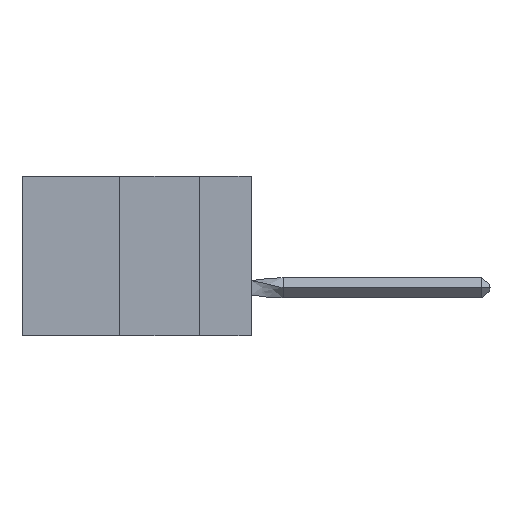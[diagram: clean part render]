
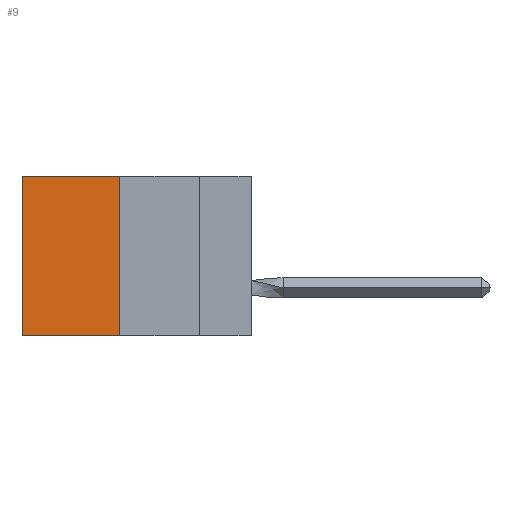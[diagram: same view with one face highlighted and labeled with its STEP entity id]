
A CAD part, left-side view. The second image highlights one B-rep face of the part: STEP entity #9.
In plain terms, the highlighted planar face has unit normal (-1, 0, 0).
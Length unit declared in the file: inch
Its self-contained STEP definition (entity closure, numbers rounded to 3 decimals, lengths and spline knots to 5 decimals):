
#9 = ADVANCED_FACE ( 'NONE', ( #1995 ), #11821, .F. ) ;
#97 = VERTEX_POINT ( 'NONE', #4743 ) ;
#1810 = CARTESIAN_POINT ( 'NONE',  ( 0.305, 0.413, -0.5 ) ) ;
#1995 = FACE_OUTER_BOUND ( 'NONE', #10964, .T. ) ;
#2162 = AXIS2_PLACEMENT_3D ( 'NONE', #10183, #5823, #2902 ) ;
#2425 = VECTOR ( 'NONE', #12045, 39.37008 ) ;
#2432 = ORIENTED_EDGE ( 'NONE', *, *, #2916, .F. ) ;
#2772 = VECTOR ( 'NONE', #9825, 39.37008 ) ;
#2902 = DIRECTION ( 'NONE',  ( 0., 0., -1. ) ) ;
#2916 = EDGE_CURVE ( 'NONE', #9484, #15254, #4434, .T. ) ;
#3051 = CARTESIAN_POINT ( 'NONE',  ( 0.305, 0.413, 0. ) ) ;
#4003 = CARTESIAN_POINT ( 'NONE',  ( 0.305, 0.413, -0.5 ) ) ;
#4434 = LINE ( 'NONE', #6071, #2425 ) ;
#4503 = CARTESIAN_POINT ( 'NONE',  ( 0.305, 0.413, 0. ) ) ;
#4509 = ORIENTED_EDGE ( 'NONE', *, *, #4709, .T. ) ;
#4709 = EDGE_CURVE ( 'NONE', #15734, #97, #6680, .T. ) ;
#4743 = CARTESIAN_POINT ( 'NONE',  ( 0.305, 0.72, -0.5 ) ) ;
#5823 = DIRECTION ( 'NONE',  ( 1., 0., 0. ) ) ;
#5915 = DIRECTION ( 'NONE',  ( 0., 1., 0. ) ) ;
#6071 = CARTESIAN_POINT ( 'NONE',  ( 0.305, 0.413, -0.5 ) ) ;
#6227 = VECTOR ( 'NONE', #6794, 39.37008 ) ;
#6680 = LINE ( 'NONE', #11145, #6227 ) ;
#6794 = DIRECTION ( 'NONE',  ( 0., 0., -1. ) ) ;
#9398 = EDGE_CURVE ( 'NONE', #9484, #15734, #13157, .T. ) ;
#9484 = VERTEX_POINT ( 'NONE', #3051 ) ;
#9825 = DIRECTION ( 'NONE',  ( 0., 1., 0. ) ) ;
#10153 = CARTESIAN_POINT ( 'NONE',  ( 0.305, 0.72, 0. ) ) ;
#10183 = CARTESIAN_POINT ( 'NONE',  ( 0.305, 0.413, -0.5 ) ) ;
#10964 = EDGE_LOOP ( 'NONE', ( #4509, #12383, #2432, #12021 ) ) ;
#11145 = CARTESIAN_POINT ( 'NONE',  ( 0.305, 0.72, -0.5 ) ) ;
#11201 = LINE ( 'NONE', #4003, #2772 ) ;
#11821 = PLANE ( 'NONE',  #2162 ) ;
#12021 = ORIENTED_EDGE ( 'NONE', *, *, #9398, .T. ) ;
#12045 = DIRECTION ( 'NONE',  ( 0., 0., -1. ) ) ;
#12383 = ORIENTED_EDGE ( 'NONE', *, *, #17757, .F. ) ;
#13157 = LINE ( 'NONE', #4503, #15901 ) ;
#15254 = VERTEX_POINT ( 'NONE', #1810 ) ;
#15734 = VERTEX_POINT ( 'NONE', #10153 ) ;
#15901 = VECTOR ( 'NONE', #5915, 39.37008 ) ;
#17757 = EDGE_CURVE ( 'NONE', #15254, #97, #11201, .T. ) ;
